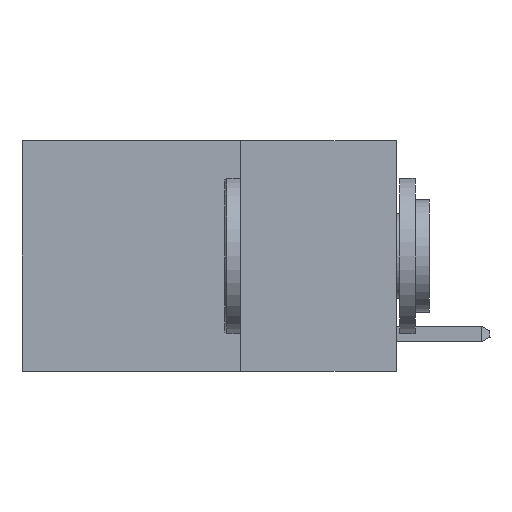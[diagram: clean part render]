
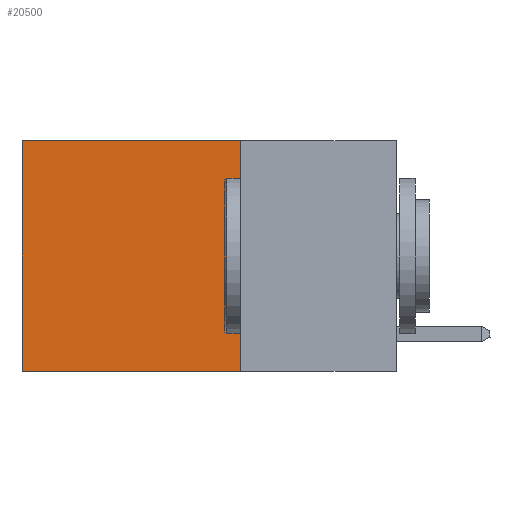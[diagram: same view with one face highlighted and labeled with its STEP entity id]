
A CAD part, left-side view. The second image highlights one B-rep face of the part: STEP entity #20500.
In plain terms, the highlighted planar face has unit normal (-1, 0, 0).
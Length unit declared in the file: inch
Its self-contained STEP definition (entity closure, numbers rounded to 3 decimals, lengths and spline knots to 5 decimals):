
#3617 = EDGE_CURVE ( 'NONE', #15932, #21363, #21355, .T. ) ;
#3627 = DIRECTION ( 'NONE',  ( 0., 0., -1. ) ) ;
#6235 = VERTEX_POINT ( 'NONE', #27711 ) ;
#6586 = DIRECTION ( 'NONE',  ( 0., 0., -1. ) ) ;
#8019 = LINE ( 'NONE', #14684, #19130 ) ;
#8832 = ORIENTED_EDGE ( 'NONE', *, *, #26675, .F. ) ;
#8892 = ORIENTED_EDGE ( 'NONE', *, *, #23613, .T. ) ;
#8927 = VECTOR ( 'NONE', #3627, 39.37008 ) ;
#10339 = CARTESIAN_POINT ( 'NONE',  ( 0.2625, 0.25, 0. ) ) ;
#10609 = LINE ( 'NONE', #12363, #23733 ) ;
#10625 = DIRECTION ( 'NONE',  ( 0., 0., -1. ) ) ;
#11768 = CARTESIAN_POINT ( 'NONE',  ( 0.2625, 0.25, -0.37 ) ) ;
#12363 = CARTESIAN_POINT ( 'NONE',  ( 0.2625, 0.25, -0.37 ) ) ;
#13265 = FACE_OUTER_BOUND ( 'NONE', #14681, .T. ) ;
#13343 = ORIENTED_EDGE ( 'NONE', *, *, #21570, .T. ) ;
#13374 = ORIENTED_EDGE ( 'NONE', *, *, #3617, .F. ) ;
#14681 = EDGE_LOOP ( 'NONE', ( #8892, #8832, #13374, #13343 ) ) ;
#14684 = CARTESIAN_POINT ( 'NONE',  ( 0.2625, 0.25, 0. ) ) ;
#15465 = CARTESIAN_POINT ( 'NONE',  ( 0.2625, 0.6, -0.37 ) ) ;
#15932 = VERTEX_POINT ( 'NONE', #24098 ) ;
#16804 = DIRECTION ( 'NONE',  ( 0., 1., 0. ) ) ;
#19128 = VERTEX_POINT ( 'NONE', #15465 ) ;
#19130 = VECTOR ( 'NONE', #16804, 39.37008 ) ;
#19459 = PLANE ( 'NONE',  #28469 ) ;
#20500 = ADVANCED_FACE ( 'NONE', ( #13265 ), #19459, .F. ) ;
#20513 = VECTOR ( 'NONE', #6586, 39.37008 ) ;
#21244 = DIRECTION ( 'NONE',  ( 0., 1., 0. ) ) ;
#21355 = LINE ( 'NONE', #10339, #8927 ) ;
#21363 = VERTEX_POINT ( 'NONE', #11768 ) ;
#21570 = EDGE_CURVE ( 'NONE', #15932, #6235, #8019, .T. ) ;
#21647 = CARTESIAN_POINT ( 'NONE',  ( 0.2625, 0.25, 0. ) ) ;
#22077 = CARTESIAN_POINT ( 'NONE',  ( 0.2625, 0.6, 0. ) ) ;
#23613 = EDGE_CURVE ( 'NONE', #6235, #19128, #27039, .T. ) ;
#23733 = VECTOR ( 'NONE', #21244, 39.37008 ) ;
#23849 = DIRECTION ( 'NONE',  ( 1., 0., 0. ) ) ;
#24098 = CARTESIAN_POINT ( 'NONE',  ( 0.2625, 0.25, 0. ) ) ;
#26675 = EDGE_CURVE ( 'NONE', #21363, #19128, #10609, .T. ) ;
#27039 = LINE ( 'NONE', #22077, #20513 ) ;
#27711 = CARTESIAN_POINT ( 'NONE',  ( 0.2625, 0.6, 0. ) ) ;
#28469 = AXIS2_PLACEMENT_3D ( 'NONE', #21647, #23849, #10625 ) ;
